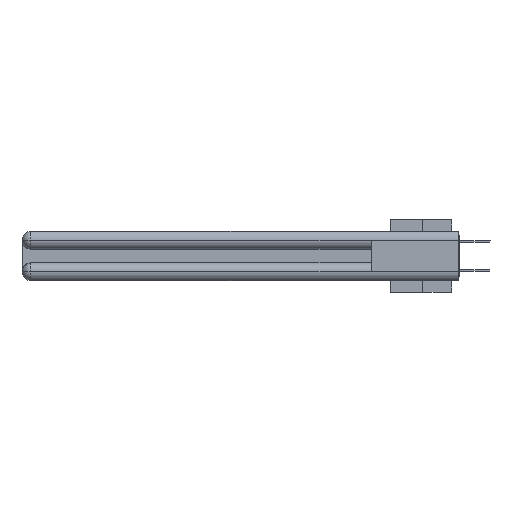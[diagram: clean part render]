
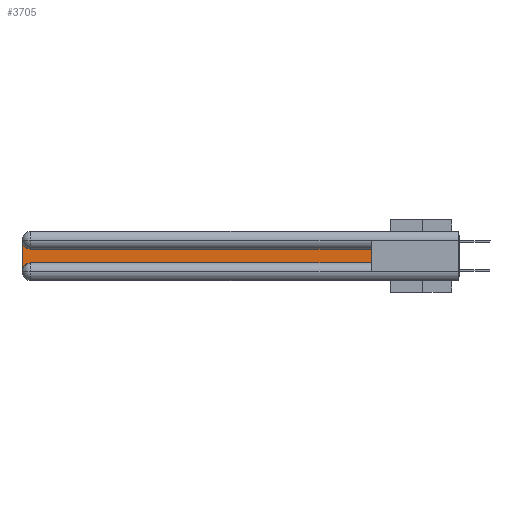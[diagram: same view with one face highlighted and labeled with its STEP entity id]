
A CAD part, left-side view. The second image highlights one B-rep face of the part: STEP entity #3705.
In plain terms, the highlighted planar face has unit normal (-1, 0, 0).
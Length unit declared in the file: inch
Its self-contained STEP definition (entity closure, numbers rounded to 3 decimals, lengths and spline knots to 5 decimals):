
#550 = CARTESIAN_POINT ( 'NONE',  ( 0.075, 3., -0.2775 ) ) ;
#1234 = ORIENTED_EDGE ( 'NONE', *, *, #28748, .T. ) ;
#1444 = LINE ( 'NONE', #21835, #14772 ) ;
#2383 = FACE_OUTER_BOUND ( 'NONE', #28570, .T. ) ;
#2750 = DIRECTION ( 'NONE',  ( 0., 0., -1. ) ) ;
#2909 = ORIENTED_EDGE ( 'NONE', *, *, #11353, .T. ) ;
#3705 = ADVANCED_FACE ( 'NONE', ( #2383 ), #37874, .F. ) ;
#3749 = EDGE_CURVE ( 'NONE', #12743, #34608, #10486, .T. ) ;
#4205 = DIRECTION ( 'NONE',  ( 0., 1., 0. ) ) ;
#5139 = VERTEX_POINT ( 'NONE', #24271 ) ;
#6979 = ORIENTED_EDGE ( 'NONE', *, *, #33689, .T. ) ;
#7177 = CIRCLE ( 'NONE', #18689, 0.06 ) ;
#7818 = VECTOR ( 'NONE', #16764, 39.37008 ) ;
#8166 = CARTESIAN_POINT ( 'NONE',  ( 0.075, 2.94, -0.2775 ) ) ;
#9709 = LINE ( 'NONE', #16711, #22029 ) ;
#10486 = LINE ( 'NONE', #13635, #37914 ) ;
#10700 = DIRECTION ( 'NONE',  ( 0., 0., -1. ) ) ;
#11353 = EDGE_CURVE ( 'NONE', #5139, #12743, #7177, .T. ) ;
#11441 = CARTESIAN_POINT ( 'NONE',  ( 0.075, 2.94, -0.0625 ) ) ;
#12146 = LINE ( 'NONE', #13881, #7818 ) ;
#12743 = VERTEX_POINT ( 'NONE', #27576 ) ;
#13635 = CARTESIAN_POINT ( 'NONE',  ( 0.075, 3., -0.2175 ) ) ;
#13660 = CARTESIAN_POINT ( 'NONE',  ( 0.075, 0.6, -0.2175 ) ) ;
#13881 = CARTESIAN_POINT ( 'NONE',  ( 0.075, 0.6, -0.2175 ) ) ;
#14772 = VECTOR ( 'NONE', #4205, 39.37008 ) ;
#14866 = DIRECTION ( 'NONE',  ( 1., 0., 0. ) ) ;
#16512 = DIRECTION ( 'NONE',  ( 1., 0., 0. ) ) ;
#16711 = CARTESIAN_POINT ( 'NONE',  ( 0.075, 0.6, -0.2175 ) ) ;
#16764 = DIRECTION ( 'NONE',  ( 0., -1., 0. ) ) ;
#18689 = AXIS2_PLACEMENT_3D ( 'NONE', #11441, #14866, #2750 ) ;
#20507 = VERTEX_POINT ( 'NONE', #13660 ) ;
#21444 = VERTEX_POINT ( 'NONE', #21517 ) ;
#21517 = CARTESIAN_POINT ( 'NONE',  ( 0.075, 0.6, -0.1225 ) ) ;
#21835 = CARTESIAN_POINT ( 'NONE',  ( 0.075, 0.6, -0.1225 ) ) ;
#22029 = VECTOR ( 'NONE', #25573, 39.37008 ) ;
#22601 = DIRECTION ( 'NONE',  ( 0., 0., -1. ) ) ;
#23139 = EDGE_CURVE ( 'NONE', #21444, #5139, #1444, .T. ) ;
#24085 = ORIENTED_EDGE ( 'NONE', *, *, #3749, .T. ) ;
#24271 = CARTESIAN_POINT ( 'NONE',  ( 0.075, 2.94, -0.1225 ) ) ;
#25375 = CARTESIAN_POINT ( 'NONE',  ( 0.075, 3., -0.1225 ) ) ;
#25573 = DIRECTION ( 'NONE',  ( 0., 0., 1. ) ) ;
#27576 = CARTESIAN_POINT ( 'NONE',  ( 0.075, 3., -0.0625 ) ) ;
#28035 = EDGE_CURVE ( 'NONE', #29189, #20507, #12146, .T. ) ;
#28294 = CARTESIAN_POINT ( 'NONE',  ( 0.075, 2.94, -0.2175 ) ) ;
#28570 = EDGE_LOOP ( 'NONE', ( #29438, #2909, #24085, #6979, #37944, #1234 ) ) ;
#28748 = EDGE_CURVE ( 'NONE', #20507, #21444, #9709, .T. ) ;
#29126 = DIRECTION ( 'NONE',  ( 1., 0., 0. ) ) ;
#29189 = VERTEX_POINT ( 'NONE', #28294 ) ;
#29438 = ORIENTED_EDGE ( 'NONE', *, *, #23139, .T. ) ;
#33689 = EDGE_CURVE ( 'NONE', #34608, #29189, #33963, .T. ) ;
#33694 = AXIS2_PLACEMENT_3D ( 'NONE', #25375, #16512, #22601 ) ;
#33963 = CIRCLE ( 'NONE', #36890, 0.06 ) ;
#34608 = VERTEX_POINT ( 'NONE', #550 ) ;
#36890 = AXIS2_PLACEMENT_3D ( 'NONE', #8166, #29126, #38321 ) ;
#37874 = PLANE ( 'NONE',  #33694 ) ;
#37914 = VECTOR ( 'NONE', #10700, 39.37008 ) ;
#37944 = ORIENTED_EDGE ( 'NONE', *, *, #28035, .T. ) ;
#38321 = DIRECTION ( 'NONE',  ( 0., 0., -1. ) ) ;
